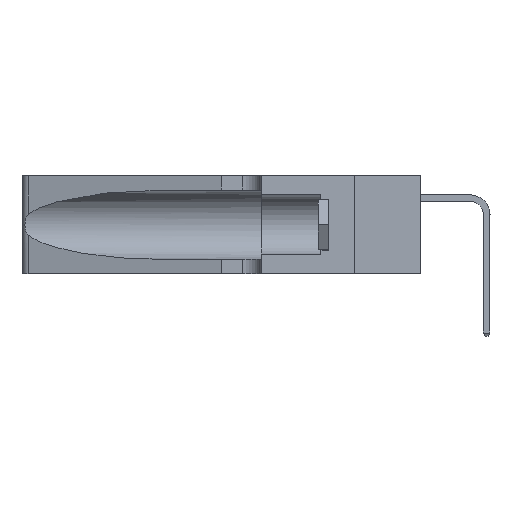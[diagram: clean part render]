
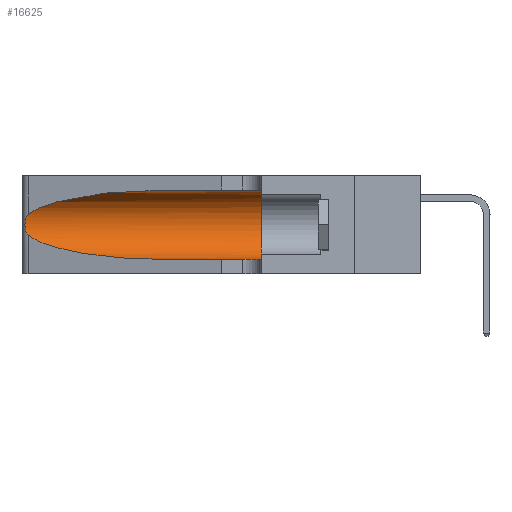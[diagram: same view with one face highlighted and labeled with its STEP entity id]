
A CAD part, left-side view. The second image highlights one B-rep face of the part: STEP entity #16625.
In plain terms, the highlighted cylindrical face has radius 3.308 mm (diameter 6.617 mm), a partial arc.
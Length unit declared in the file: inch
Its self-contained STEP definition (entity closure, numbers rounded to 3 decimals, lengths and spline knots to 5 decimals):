
#192 = CARTESIAN_POINT ( 'NONE',  ( 0.25555, 1.22993, 0.14849 ) ) ;
#719 = VECTOR ( 'NONE', #7427, 39.37008 ) ;
#841 = EDGE_LOOP ( 'NONE', ( #26020, #3356, #15817, #19135, #12970, #5734 ) ) ;
#2775 = LINE ( 'NONE', #40110, #719 ) ;
#3171 = EDGE_CURVE ( 'NONE', #30839, #12183, #29021, .T. ) ;
#3356 = ORIENTED_EDGE ( 'NONE', *, *, #3171, .T. ) ;
#3367 = CARTESIAN_POINT ( 'NONE',  ( 0.25555, 1.22994, 0.2215 ) ) ;
#3500 = DIRECTION ( 'NONE',  ( 0., -1., 0. ) ) ;
#4030 = CARTESIAN_POINT ( 'NONE',  ( 0.25487, 1.22718, 0.14631 ) ) ;
#5734 = ORIENTED_EDGE ( 'NONE', *, *, #29044, .F. ) ;
#6070 =( BOUNDED_CURVE ( )  B_SPLINE_CURVE ( 3, ( #4030, #10860, #40320, #20814 ),
 .UNSPECIFIED., .F., .T. ) 
 B_SPLINE_CURVE_WITH_KNOTS ( ( 4, 4 ),
 ( 3.44316, 4.71239 ),
 .UNSPECIFIED. ) 
 CURVE ( )  GEOMETRIC_REPRESENTATION_ITEM ( )  RATIONAL_B_SPLINE_CURVE ( ( 1., 0.87, 0.87, 1. ) ) 
 REPRESENTATION_ITEM ( '' )  );
#6379 = DIRECTION ( 'NONE',  ( 0., -1., 0. ) ) ;
#6417 = CARTESIAN_POINT ( 'NONE',  ( 0.25487, 1.22718, 0.22369 ) ) ;
#6708 = CARTESIAN_POINT ( 'NONE',  ( 0.25787, 1.23484, 0.2124 ) ) ;
#7427 = DIRECTION ( 'NONE',  ( 0., -1., 0. ) ) ;
#8555 = EDGE_CURVE ( 'NONE', #12183, #20538, #6070, .T. ) ;
#9158 = CARTESIAN_POINT ( 'NONE',  ( 0.1305, 0.35, 0.185 ) ) ;
#9453 = CYLINDRICAL_SURFACE ( 'NONE', #39141, 0.13025 ) ;
#9714 = EDGE_CURVE ( 'NONE', #20538, #25545, #2775, .T. ) ;
#10043 = CARTESIAN_POINT ( 'NONE',  ( 0.26018, 1.23835, 0.19895 ) ) ;
#10344 = CARTESIAN_POINT ( 'NONE',  ( 0.1305, 0.72297, 0.05475 ) ) ;
#10608 = EDGE_CURVE ( 'NONE', #39457, #25545, #42185, .T. ) ;
#10860 = CARTESIAN_POINT ( 'NONE',  ( 0.2373, 1.15595, 0.08982 ) ) ;
#12183 = VERTEX_POINT ( 'NONE', #17013 ) ;
#12512 = DIRECTION ( 'NONE',  ( 0., 0., 1. ) ) ;
#12970 = ORIENTED_EDGE ( 'NONE', *, *, #10608, .F. ) ;
#13382 = CARTESIAN_POINT ( 'NONE',  ( 0.26075, 1.23896, 0.178 ) ) ;
#14462 = AXIS2_PLACEMENT_3D ( 'NONE', #9158, #32149, #12512 ) ;
#15817 = ORIENTED_EDGE ( 'NONE', *, *, #8555, .T. ) ;
#16240 = CARTESIAN_POINT ( 'NONE',  ( 0.2373, 1.15595, 0.28018 ) ) ;
#16625 = ADVANCED_FACE ( 'NONE', ( #20325 ), #9453, .F. ) ;
#16687 = CARTESIAN_POINT ( 'NONE',  ( 0.25856, 1.23593, 0.16098 ) ) ;
#17013 = CARTESIAN_POINT ( 'NONE',  ( 0.25487, 1.22718, 0.14631 ) ) ;
#17535 = VERTEX_POINT ( 'NONE', #40281 ) ;
#18428 = CARTESIAN_POINT ( 'NONE',  ( 0.1305, 0.35, 0.31525 ) ) ;
#19135 = ORIENTED_EDGE ( 'NONE', *, *, #9714, .T. ) ;
#19845 =( BOUNDED_CURVE ( )  B_SPLINE_CURVE ( 3, ( #29287, #22719, #16240, #39108 ),
 .UNSPECIFIED., .F., .F. ) 
 B_SPLINE_CURVE_WITH_KNOTS ( ( 4, 4 ),
 ( 1.5708, 2.84003 ),
 .UNSPECIFIED. ) 
 CURVE ( )  GEOMETRIC_REPRESENTATION_ITEM ( )  RATIONAL_B_SPLINE_CURVE ( ( 1., 0.87, 0.87, 1. ) ) 
 REPRESENTATION_ITEM ( '' )  );
#20009 = CARTESIAN_POINT ( 'NONE',  ( 0.25639, 1.23186, 0.15144 ) ) ;
#20039 = LINE ( 'NONE', #23282, #37372 ) ;
#20325 = FACE_OUTER_BOUND ( 'NONE', #841, .T. ) ;
#20538 = VERTEX_POINT ( 'NONE', #10344 ) ;
#20814 = CARTESIAN_POINT ( 'NONE',  ( 0.1305, 0.72297, 0.05475 ) ) ;
#22719 = CARTESIAN_POINT ( 'NONE',  ( 0.18966, 0.96281, 0.31525 ) ) ;
#22835 = CARTESIAN_POINT ( 'NONE',  ( 0.1305, 1.61858, 0.185 ) ) ;
#23141 = CARTESIAN_POINT ( 'NONE',  ( 0.25639, 1.23184, 0.21858 ) ) ;
#23282 = CARTESIAN_POINT ( 'NONE',  ( 0.1305, 1.61858, 0.31525 ) ) ;
#23289 = CARTESIAN_POINT ( 'NONE',  ( 0.25487, 1.22718, 0.14631 ) ) ;
#25545 = VERTEX_POINT ( 'NONE', #35223 ) ;
#26020 = ORIENTED_EDGE ( 'NONE', *, *, #28958, .T. ) ;
#26107 = DIRECTION ( 'NONE',  ( 0., 0., -1. ) ) ;
#28958 = EDGE_CURVE ( 'NONE', #17535, #30839, #19845, .T. ) ;
#29021 = B_SPLINE_CURVE_WITH_KNOTS ( 'NONE', 3,
 ( #32847, #3367, #23141, #6708, #29706, #10043, #32983, #13382, #36270, #16687, #39530, #20009, #192, #23289 ),
 .UNSPECIFIED., .F., .F.,
 ( 4, 2, 2, 2, 2, 2, 4 ),
 ( 0., 0.00027, 0.00053, 0.00107, 0.0016, 0.00187, 0.00214 ),
 .UNSPECIFIED. ) ;
#29044 = EDGE_CURVE ( 'NONE', #17535, #39457, #20039, .T. ) ;
#29287 = CARTESIAN_POINT ( 'NONE',  ( 0.1305, 0.72297, 0.31525 ) ) ;
#29706 = CARTESIAN_POINT ( 'NONE',  ( 0.25854, 1.2359, 0.20912 ) ) ;
#30839 = VERTEX_POINT ( 'NONE', #6417 ) ;
#32149 = DIRECTION ( 'NONE',  ( 0., 1., 0. ) ) ;
#32847 = CARTESIAN_POINT ( 'NONE',  ( 0.25487, 1.22718, 0.22369 ) ) ;
#32983 = CARTESIAN_POINT ( 'NONE',  ( 0.26075, 1.23896, 0.19203 ) ) ;
#35223 = CARTESIAN_POINT ( 'NONE',  ( 0.1305, 0.35, 0.05475 ) ) ;
#36270 = CARTESIAN_POINT ( 'NONE',  ( 0.26017, 1.23833, 0.17102 ) ) ;
#37372 = VECTOR ( 'NONE', #3500, 39.37008 ) ;
#39108 = CARTESIAN_POINT ( 'NONE',  ( 0.25487, 1.22718, 0.22369 ) ) ;
#39141 = AXIS2_PLACEMENT_3D ( 'NONE', #22835, #6379, #26107 ) ;
#39457 = VERTEX_POINT ( 'NONE', #18428 ) ;
#39530 = CARTESIAN_POINT ( 'NONE',  ( 0.25789, 1.23486, 0.15765 ) ) ;
#40110 = CARTESIAN_POINT ( 'NONE',  ( 0.1305, 1.61858, 0.05475 ) ) ;
#40281 = CARTESIAN_POINT ( 'NONE',  ( 0.1305, 0.72297, 0.31525 ) ) ;
#40320 = CARTESIAN_POINT ( 'NONE',  ( 0.18966, 0.96281, 0.05475 ) ) ;
#42185 = CIRCLE ( 'NONE', #14462, 0.13025 ) ;
